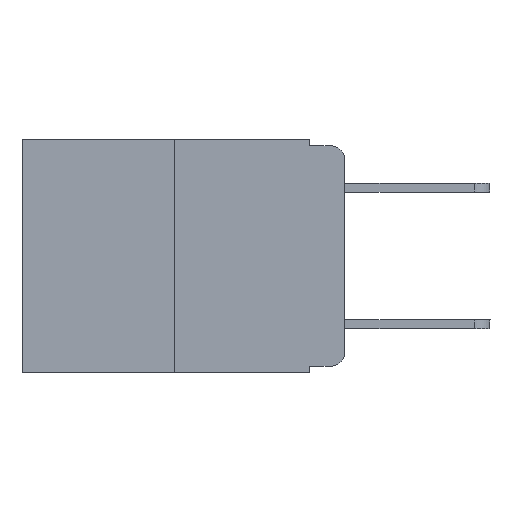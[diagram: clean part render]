
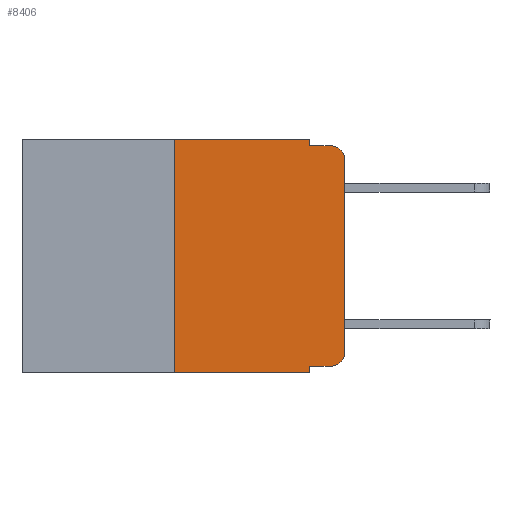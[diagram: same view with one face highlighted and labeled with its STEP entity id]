
A CAD part, left-side view. The second image highlights one B-rep face of the part: STEP entity #8406.
In plain terms, the highlighted planar face has unit normal (-1, 0, 0).
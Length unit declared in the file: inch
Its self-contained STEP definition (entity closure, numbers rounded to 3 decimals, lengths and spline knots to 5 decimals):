
#278 = VERTEX_POINT ( 'NONE', #14765 ) ;
#280 = EDGE_CURVE ( 'NONE', #6762, #278, #14954, .T. ) ;
#296 = LINE ( 'NONE', #15344, #12205 ) ;
#316 = CARTESIAN_POINT ( 'NONE',  ( 0., 0.051, 0. ) ) ;
#352 = VECTOR ( 'NONE', #1088, 39.37008 ) ;
#403 = VECTOR ( 'NONE', #6156, 39.37008 ) ;
#612 = VECTOR ( 'NONE', #10939, 39.37008 ) ;
#732 = EDGE_CURVE ( 'NONE', #8894, #6762, #7351, .T. ) ;
#1088 = DIRECTION ( 'NONE',  ( 0., -1., 0. ) ) ;
#1219 = VERTEX_POINT ( 'NONE', #3470 ) ;
#1441 = EDGE_CURVE ( 'NONE', #1219, #11345, #2780, .T. ) ;
#1753 = EDGE_CURVE ( 'NONE', #7339, #13935, #296, .T. ) ;
#1947 = CARTESIAN_POINT ( 'NONE',  ( 0., 0., -0.313 ) ) ;
#1984 = AXIS2_PLACEMENT_3D ( 'NONE', #14372, #4055, #9243 ) ;
#2051 = LINE ( 'NONE', #16717, #10903 ) ;
#2472 = CARTESIAN_POINT ( 'NONE',  ( 0., 0.051, 0. ) ) ;
#2602 = ORIENTED_EDGE ( 'NONE', *, *, #5908, .F. ) ;
#2677 = CARTESIAN_POINT ( 'NONE',  ( 0., 0.473, 0. ) ) ;
#2765 = VERTEX_POINT ( 'NONE', #1947 ) ;
#2780 = CIRCLE ( 'NONE', #4530, 0.02 ) ;
#2804 = CARTESIAN_POINT ( 'NONE',  ( 0., 0.051, 0. ) ) ;
#3008 = LINE ( 'NONE', #316, #13928 ) ;
#3271 = CARTESIAN_POINT ( 'NONE',  ( 0., 0.02, -0.01 ) ) ;
#3470 = CARTESIAN_POINT ( 'NONE',  ( 0., 0., -0.03 ) ) ;
#4055 = DIRECTION ( 'NONE',  ( -1., 0., 0. ) ) ;
#4128 = ORIENTED_EDGE ( 'NONE', *, *, #1753, .T. ) ;
#4202 = VECTOR ( 'NONE', #8205, 39.37008 ) ;
#4351 = EDGE_LOOP ( 'NONE', ( #4495, #12009, #14115, #14805, #17055, #12353, #4128, #2602, #15974, #5657 ) ) ;
#4495 = ORIENTED_EDGE ( 'NONE', *, *, #4640, .T. ) ;
#4526 = EDGE_CURVE ( 'NONE', #12200, #15167, #2051, .T. ) ;
#4530 = AXIS2_PLACEMENT_3D ( 'NONE', #15955, #10775, #8117 ) ;
#4640 = EDGE_CURVE ( 'NONE', #2765, #1219, #16677, .T. ) ;
#4700 = AXIS2_PLACEMENT_3D ( 'NONE', #2677, #7922, #17019 ) ;
#4918 = EDGE_CURVE ( 'NONE', #278, #11345, #5927, .T. ) ;
#5467 = DIRECTION ( 'NONE',  ( 0., 0., -1. ) ) ;
#5657 = ORIENTED_EDGE ( 'NONE', *, *, #8208, .T. ) ;
#5716 = CARTESIAN_POINT ( 'NONE',  ( 0., 0.25, 0. ) ) ;
#5908 = EDGE_CURVE ( 'NONE', #12200, #13935, #3008, .T. ) ;
#5927 = LINE ( 'NONE', #16191, #612 ) ;
#6156 = DIRECTION ( 'NONE',  ( 0., 0., 1. ) ) ;
#6420 = CARTESIAN_POINT ( 'NONE',  ( 0., 0.25, -0.343 ) ) ;
#6762 = VERTEX_POINT ( 'NONE', #2472 ) ;
#6896 = LINE ( 'NONE', #13311, #4202 ) ;
#7339 = VERTEX_POINT ( 'NONE', #6420 ) ;
#7351 = LINE ( 'NONE', #9014, #352 ) ;
#7922 = DIRECTION ( 'NONE',  ( 1., 0., 0. ) ) ;
#8054 = DIRECTION ( 'NONE',  ( 0., 0., -1. ) ) ;
#8117 = DIRECTION ( 'NONE',  ( 0., 0., -1. ) ) ;
#8122 = CARTESIAN_POINT ( 'NONE',  ( 0., 0.051, -0.343 ) ) ;
#8205 = DIRECTION ( 'NONE',  ( 0., 0., 1. ) ) ;
#8208 = EDGE_CURVE ( 'NONE', #15167, #2765, #16801, .T. ) ;
#8406 = ADVANCED_FACE ( 'NONE', ( #13048 ), #14412, .F. ) ;
#8894 = VERTEX_POINT ( 'NONE', #5716 ) ;
#9014 = CARTESIAN_POINT ( 'NONE',  ( 0., 0.473, 0. ) ) ;
#9243 = DIRECTION ( 'NONE',  ( 0., 0., -1. ) ) ;
#9524 = CARTESIAN_POINT ( 'NONE',  ( 0., 0.02, -0.333 ) ) ;
#10216 = DIRECTION ( 'NONE',  ( 0., -1., 0. ) ) ;
#10775 = DIRECTION ( 'NONE',  ( -1., 0., 0. ) ) ;
#10903 = VECTOR ( 'NONE', #10216, 39.37008 ) ;
#10939 = DIRECTION ( 'NONE',  ( 0., -1., 0. ) ) ;
#11345 = VERTEX_POINT ( 'NONE', #3271 ) ;
#11404 = CARTESIAN_POINT ( 'NONE',  ( 0., 0., 0. ) ) ;
#12009 = ORIENTED_EDGE ( 'NONE', *, *, #1441, .T. ) ;
#12200 = VERTEX_POINT ( 'NONE', #16996 ) ;
#12205 = VECTOR ( 'NONE', #14015, 39.37008 ) ;
#12353 = ORIENTED_EDGE ( 'NONE', *, *, #16975, .F. ) ;
#13048 = FACE_OUTER_BOUND ( 'NONE', #4351, .T. ) ;
#13311 = CARTESIAN_POINT ( 'NONE',  ( 0., 0.25, 0. ) ) ;
#13928 = VECTOR ( 'NONE', #5467, 39.37008 ) ;
#13935 = VERTEX_POINT ( 'NONE', #8122 ) ;
#14015 = DIRECTION ( 'NONE',  ( 0., -1., 0. ) ) ;
#14115 = ORIENTED_EDGE ( 'NONE', *, *, #4918, .F. ) ;
#14372 = CARTESIAN_POINT ( 'NONE',  ( 0., 0.02, -0.313 ) ) ;
#14412 = PLANE ( 'NONE',  #4700 ) ;
#14765 = CARTESIAN_POINT ( 'NONE',  ( 0., 0.051, -0.01 ) ) ;
#14805 = ORIENTED_EDGE ( 'NONE', *, *, #280, .F. ) ;
#14954 = LINE ( 'NONE', #2804, #16641 ) ;
#15167 = VERTEX_POINT ( 'NONE', #9524 ) ;
#15344 = CARTESIAN_POINT ( 'NONE',  ( 0., 0.473, -0.343 ) ) ;
#15955 = CARTESIAN_POINT ( 'NONE',  ( 0., 0.02, -0.03 ) ) ;
#15974 = ORIENTED_EDGE ( 'NONE', *, *, #4526, .T. ) ;
#16191 = CARTESIAN_POINT ( 'NONE',  ( 0., 0.051, -0.01 ) ) ;
#16641 = VECTOR ( 'NONE', #8054, 39.37008 ) ;
#16677 = LINE ( 'NONE', #11404, #403 ) ;
#16717 = CARTESIAN_POINT ( 'NONE',  ( 0., 0.051, -0.333 ) ) ;
#16801 = CIRCLE ( 'NONE', #1984, 0.02 ) ;
#16975 = EDGE_CURVE ( 'NONE', #7339, #8894, #6896, .T. ) ;
#16996 = CARTESIAN_POINT ( 'NONE',  ( 0., 0.051, -0.333 ) ) ;
#17019 = DIRECTION ( 'NONE',  ( 0., 0., -1. ) ) ;
#17055 = ORIENTED_EDGE ( 'NONE', *, *, #732, .F. ) ;
